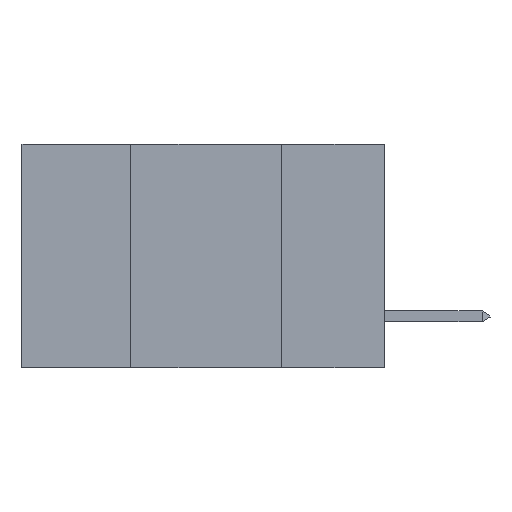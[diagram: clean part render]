
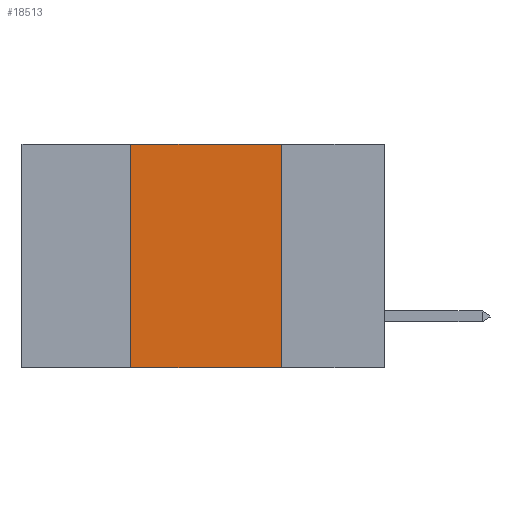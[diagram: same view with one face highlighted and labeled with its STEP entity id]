
A CAD part, left-side view. The second image highlights one B-rep face of the part: STEP entity #18513.
In plain terms, the highlighted planar face has unit normal (-1, 0, 0).
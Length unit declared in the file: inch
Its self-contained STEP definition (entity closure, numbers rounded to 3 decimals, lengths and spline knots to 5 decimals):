
#9325 = CARTESIAN_POINT ( 'NONE',  ( 0., 0.17, 0. ) ) ;
#9497 = DIRECTION ( 'NONE',  ( 0., 0., -1. ) ) ;
#9969 = DIRECTION ( 'NONE',  ( 1., 0., 0. ) ) ;
#10263 = ORIENTED_EDGE ( 'NONE', *, *, #30862, .F. ) ;
#12579 = LINE ( 'NONE', #37685, #25149 ) ;
#14659 = VERTEX_POINT ( 'NONE', #19314 ) ;
#15729 = LINE ( 'NONE', #37813, #27102 ) ;
#16758 = VECTOR ( 'NONE', #9497, 39.37008 ) ;
#17853 = DIRECTION ( 'NONE',  ( 0., -1., 0. ) ) ;
#18000 = VERTEX_POINT ( 'NONE', #44709 ) ;
#18513 = ADVANCED_FACE ( 'NONE', ( #39577 ), #40492, .F. ) ;
#19314 = CARTESIAN_POINT ( 'NONE',  ( 0., 0.42, 0. ) ) ;
#20374 = LINE ( 'NONE', #9325, #16758 ) ;
#22695 = DIRECTION ( 'NONE',  ( 0., -1., 0. ) ) ;
#22915 = AXIS2_PLACEMENT_3D ( 'NONE', #40810, #9969, #32784 ) ;
#24321 = EDGE_CURVE ( 'NONE', #40399, #35060, #15729, .T. ) ;
#25149 = VECTOR ( 'NONE', #41366, 39.37008 ) ;
#27019 = EDGE_LOOP ( 'NONE', ( #10263, #28199, #30327, #35566 ) ) ;
#27102 = VECTOR ( 'NONE', #22695, 39.37008 ) ;
#28199 = ORIENTED_EDGE ( 'NONE', *, *, #34119, .F. ) ;
#29247 = CARTESIAN_POINT ( 'NONE',  ( 0., 0.6, 0. ) ) ;
#30327 = ORIENTED_EDGE ( 'NONE', *, *, #40544, .F. ) ;
#30862 = EDGE_CURVE ( 'NONE', #18000, #35060, #20374, .T. ) ;
#32784 = DIRECTION ( 'NONE',  ( 0., 0., -1. ) ) ;
#33000 = CARTESIAN_POINT ( 'NONE',  ( 0., 0.42, -0.37 ) ) ;
#34119 = EDGE_CURVE ( 'NONE', #14659, #18000, #36127, .T. ) ;
#35060 = VERTEX_POINT ( 'NONE', #42791 ) ;
#35566 = ORIENTED_EDGE ( 'NONE', *, *, #24321, .T. ) ;
#36127 = LINE ( 'NONE', #29247, #45074 ) ;
#37685 = CARTESIAN_POINT ( 'NONE',  ( 0., 0.42, 0. ) ) ;
#37813 = CARTESIAN_POINT ( 'NONE',  ( 0., 0.6, -0.37 ) ) ;
#39577 = FACE_OUTER_BOUND ( 'NONE', #27019, .T. ) ;
#40399 = VERTEX_POINT ( 'NONE', #33000 ) ;
#40492 = PLANE ( 'NONE',  #22915 ) ;
#40544 = EDGE_CURVE ( 'NONE', #40399, #14659, #12579, .T. ) ;
#40810 = CARTESIAN_POINT ( 'NONE',  ( 0., 0.6, 0. ) ) ;
#41366 = DIRECTION ( 'NONE',  ( 0., 0., 1. ) ) ;
#42791 = CARTESIAN_POINT ( 'NONE',  ( 0., 0.17, -0.37 ) ) ;
#44709 = CARTESIAN_POINT ( 'NONE',  ( 0., 0.17, 0. ) ) ;
#45074 = VECTOR ( 'NONE', #17853, 39.37008 ) ;
